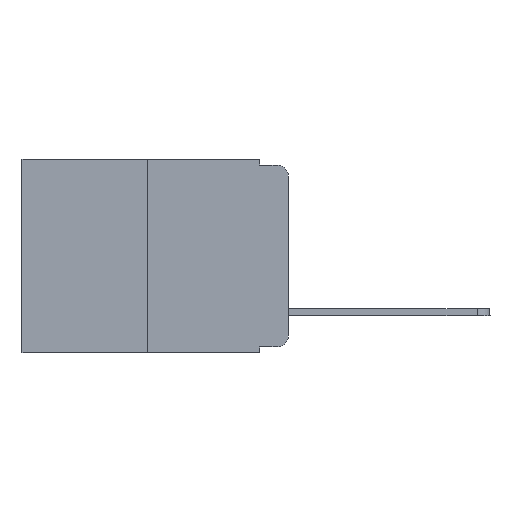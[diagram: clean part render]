
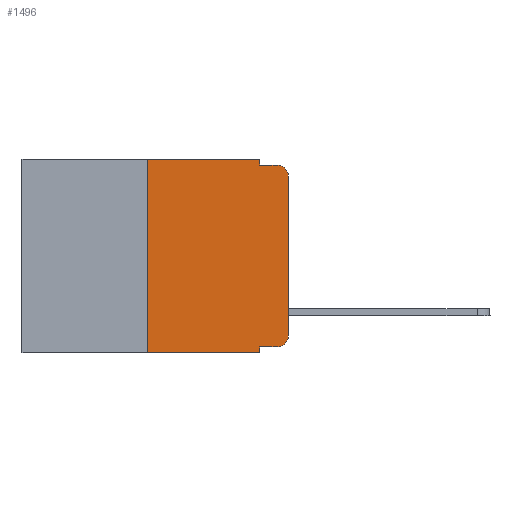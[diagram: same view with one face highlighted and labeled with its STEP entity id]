
A CAD part, left-side view. The second image highlights one B-rep face of the part: STEP entity #1496.
In plain terms, the highlighted planar face has unit normal (-1, 0, 0).
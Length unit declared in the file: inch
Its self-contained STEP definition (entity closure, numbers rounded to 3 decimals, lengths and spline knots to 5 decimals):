
#45 = DIRECTION ( 'NONE',  ( -1., 0., 0. ) ) ;
#65 = EDGE_CURVE ( 'NONE', #7962, #81, #1898, .T. ) ;
#81 = VERTEX_POINT ( 'NONE', #6741 ) ;
#212 = ORIENTED_EDGE ( 'NONE', *, *, #8405, .F. ) ;
#253 = DIRECTION ( 'NONE',  ( 0., -1., 0. ) ) ;
#266 = CARTESIAN_POINT ( 'NONE',  ( 0., 0.051, -0.343 ) ) ;
#364 = VERTEX_POINT ( 'NONE', #3347 ) ;
#464 = FACE_OUTER_BOUND ( 'NONE', #7685, .T. ) ;
#468 = AXIS2_PLACEMENT_3D ( 'NONE', #8663, #4676, #9083 ) ;
#658 = EDGE_CURVE ( 'NONE', #364, #7922, #7989, .T. ) ;
#724 = EDGE_CURVE ( 'NONE', #4832, #7962, #4791, .T. ) ;
#802 = ORIENTED_EDGE ( 'NONE', *, *, #889, .F. ) ;
#889 = EDGE_CURVE ( 'NONE', #3100, #5332, #3394, .T. ) ;
#914 = VECTOR ( 'NONE', #253, 39.37008 ) ;
#990 = CARTESIAN_POINT ( 'NONE',  ( 0., 0.051, -0.01 ) ) ;
#999 = ORIENTED_EDGE ( 'NONE', *, *, #5501, .T. ) ;
#1225 = CARTESIAN_POINT ( 'NONE',  ( 0., 0.051, 0. ) ) ;
#1334 = DIRECTION ( 'NONE',  ( 0., 0., 1. ) ) ;
#1433 = PLANE ( 'NONE',  #468 ) ;
#1464 = CARTESIAN_POINT ( 'NONE',  ( 0., 0., 0. ) ) ;
#1496 = ADVANCED_FACE ( 'NONE', ( #464 ), #1433, .F. ) ;
#1544 = CARTESIAN_POINT ( 'NONE',  ( 0., 0.25, -0.343 ) ) ;
#1545 = VECTOR ( 'NONE', #1334, 39.37008 ) ;
#1898 = LINE ( 'NONE', #1464, #8111 ) ;
#2018 = VECTOR ( 'NONE', #5200, 39.37008 ) ;
#2078 = CARTESIAN_POINT ( 'NONE',  ( 0., 0.25, 0. ) ) ;
#2121 = EDGE_CURVE ( 'NONE', #9406, #2654, #5203, .T. ) ;
#2613 = LINE ( 'NONE', #7661, #6637 ) ;
#2654 = VERTEX_POINT ( 'NONE', #990 ) ;
#2884 = ORIENTED_EDGE ( 'NONE', *, *, #2121, .F. ) ;
#2896 = ORIENTED_EDGE ( 'NONE', *, *, #65, .T. ) ;
#3100 = VERTEX_POINT ( 'NONE', #1544 ) ;
#3161 = EDGE_CURVE ( 'NONE', #2654, #4388, #5415, .T. ) ;
#3209 = CARTESIAN_POINT ( 'NONE',  ( 0., 0.02, -0.333 ) ) ;
#3265 = CARTESIAN_POINT ( 'NONE',  ( 0., 0.051, 0. ) ) ;
#3301 = LINE ( 'NONE', #4472, #2018 ) ;
#3347 = CARTESIAN_POINT ( 'NONE',  ( 0., 0.051, -0.333 ) ) ;
#3394 = LINE ( 'NONE', #2078, #1545 ) ;
#3442 = DIRECTION ( 'NONE',  ( 0., 0., -1. ) ) ;
#3534 = CIRCLE ( 'NONE', #5863, 0.02 ) ;
#4388 = VERTEX_POINT ( 'NONE', #5541 ) ;
#4449 = DIRECTION ( 'NONE',  ( 0., -1., 0. ) ) ;
#4472 = CARTESIAN_POINT ( 'NONE',  ( 0., 0.473, -0.343 ) ) ;
#4676 = DIRECTION ( 'NONE',  ( 1., 0., 0. ) ) ;
#4685 = VECTOR ( 'NONE', #5465, 39.37008 ) ;
#4757 = CARTESIAN_POINT ( 'NONE',  ( 0., 0., -0.313 ) ) ;
#4791 = CIRCLE ( 'NONE', #6017, 0.02 ) ;
#4832 = VERTEX_POINT ( 'NONE', #3209 ) ;
#4966 = DIRECTION ( 'NONE',  ( 0., 0., -1. ) ) ;
#5107 = EDGE_CURVE ( 'NONE', #81, #4388, #3534, .T. ) ;
#5200 = DIRECTION ( 'NONE',  ( 0., -1., 0. ) ) ;
#5203 = LINE ( 'NONE', #9349, #9552 ) ;
#5332 = VERTEX_POINT ( 'NONE', #5785 ) ;
#5415 = LINE ( 'NONE', #8993, #914 ) ;
#5465 = DIRECTION ( 'NONE',  ( 0., 0., -1. ) ) ;
#5501 = EDGE_CURVE ( 'NONE', #3100, #7922, #3301, .T. ) ;
#5512 = DIRECTION ( 'NONE',  ( 0., -1., 0. ) ) ;
#5541 = CARTESIAN_POINT ( 'NONE',  ( 0., 0.02, -0.01 ) ) ;
#5785 = CARTESIAN_POINT ( 'NONE',  ( 0., 0.25, 0. ) ) ;
#5849 = CARTESIAN_POINT ( 'NONE',  ( 0., 0.473, 0. ) ) ;
#5863 = AXIS2_PLACEMENT_3D ( 'NONE', #7477, #45, #8853 ) ;
#6017 = AXIS2_PLACEMENT_3D ( 'NONE', #7742, #9316, #3442 ) ;
#6409 = ORIENTED_EDGE ( 'NONE', *, *, #3161, .F. ) ;
#6637 = VECTOR ( 'NONE', #5512, 39.37008 ) ;
#6741 = CARTESIAN_POINT ( 'NONE',  ( 0., 0., -0.03 ) ) ;
#7477 = CARTESIAN_POINT ( 'NONE',  ( 0., 0.02, -0.03 ) ) ;
#7661 = CARTESIAN_POINT ( 'NONE',  ( 0., 0.051, -0.333 ) ) ;
#7672 = LINE ( 'NONE', #5849, #9393 ) ;
#7685 = EDGE_LOOP ( 'NONE', ( #2896, #7881, #6409, #2884, #212, #802, #999, #9061, #9396, #8617 ) ) ;
#7742 = CARTESIAN_POINT ( 'NONE',  ( 0., 0.02, -0.313 ) ) ;
#7881 = ORIENTED_EDGE ( 'NONE', *, *, #5107, .T. ) ;
#7922 = VERTEX_POINT ( 'NONE', #266 ) ;
#7962 = VERTEX_POINT ( 'NONE', #4757 ) ;
#7989 = LINE ( 'NONE', #3265, #4685 ) ;
#8111 = VECTOR ( 'NONE', #8893, 39.37008 ) ;
#8405 = EDGE_CURVE ( 'NONE', #5332, #9406, #7672, .T. ) ;
#8617 = ORIENTED_EDGE ( 'NONE', *, *, #724, .T. ) ;
#8663 = CARTESIAN_POINT ( 'NONE',  ( 0., 0.473, 0. ) ) ;
#8853 = DIRECTION ( 'NONE',  ( 0., 0., -1. ) ) ;
#8893 = DIRECTION ( 'NONE',  ( 0., 0., 1. ) ) ;
#8993 = CARTESIAN_POINT ( 'NONE',  ( 0., 0.051, -0.01 ) ) ;
#9061 = ORIENTED_EDGE ( 'NONE', *, *, #658, .F. ) ;
#9083 = DIRECTION ( 'NONE',  ( 0., 0., -1. ) ) ;
#9309 = EDGE_CURVE ( 'NONE', #364, #4832, #2613, .T. ) ;
#9316 = DIRECTION ( 'NONE',  ( -1., 0., 0. ) ) ;
#9349 = CARTESIAN_POINT ( 'NONE',  ( 0., 0.051, 0. ) ) ;
#9393 = VECTOR ( 'NONE', #4449, 39.37008 ) ;
#9396 = ORIENTED_EDGE ( 'NONE', *, *, #9309, .T. ) ;
#9406 = VERTEX_POINT ( 'NONE', #1225 ) ;
#9552 = VECTOR ( 'NONE', #4966, 39.37008 ) ;
